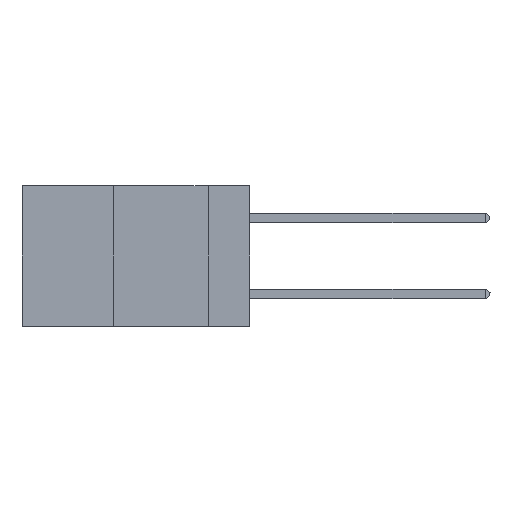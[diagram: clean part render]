
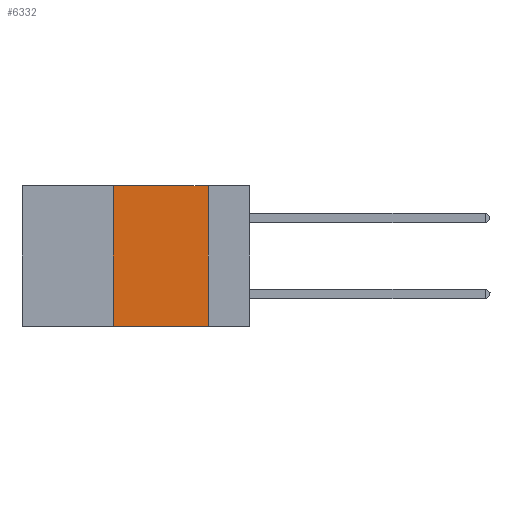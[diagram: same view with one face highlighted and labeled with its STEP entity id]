
A CAD part, left-side view. The second image highlights one B-rep face of the part: STEP entity #6332.
In plain terms, the highlighted planar face has unit normal (-1, 0, 0).
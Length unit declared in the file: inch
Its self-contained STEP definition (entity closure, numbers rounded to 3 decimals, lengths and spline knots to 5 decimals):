
#1540 = EDGE_CURVE ( 'NONE', #17693, #9061, #7145, .T. ) ;
#1716 = LINE ( 'NONE', #33998, #30821 ) ;
#2423 = VECTOR ( 'NONE', #25218, 39.37008 ) ;
#3049 = ORIENTED_EDGE ( 'NONE', *, *, #26859, .F. ) ;
#4459 = LINE ( 'NONE', #15882, #4602 ) ;
#4602 = VECTOR ( 'NONE', #21178, 39.37008 ) ;
#4839 = CARTESIAN_POINT ( 'NONE',  ( 0., 0.6, -0.37 ) ) ;
#5854 = CARTESIAN_POINT ( 'NONE',  ( 0., 0.6, 0. ) ) ;
#5883 = DIRECTION ( 'NONE',  ( 0., 0., -1. ) ) ;
#6332 = ADVANCED_FACE ( 'NONE', ( #7829 ), #34083, .F. ) ;
#7145 = LINE ( 'NONE', #4839, #18668 ) ;
#7829 = FACE_OUTER_BOUND ( 'NONE', #8242, .T. ) ;
#8237 = CARTESIAN_POINT ( 'NONE',  ( 0., 0.11, -0.37 ) ) ;
#8242 = EDGE_LOOP ( 'NONE', ( #3049, #34082, #18539, #13678 ) ) ;
#9061 = VERTEX_POINT ( 'NONE', #8237 ) ;
#10597 = AXIS2_PLACEMENT_3D ( 'NONE', #31429, #15391, #5883 ) ;
#12482 = DIRECTION ( 'NONE',  ( 0., 0., -1. ) ) ;
#13678 = ORIENTED_EDGE ( 'NONE', *, *, #1540, .T. ) ;
#15391 = DIRECTION ( 'NONE',  ( 1., 0., 0. ) ) ;
#15882 = CARTESIAN_POINT ( 'NONE',  ( 0., 0.36, 0. ) ) ;
#17554 = EDGE_CURVE ( 'NONE', #17693, #19803, #4459, .T. ) ;
#17693 = VERTEX_POINT ( 'NONE', #22048 ) ;
#18539 = ORIENTED_EDGE ( 'NONE', *, *, #17554, .F. ) ;
#18668 = VECTOR ( 'NONE', #20193, 39.37008 ) ;
#19595 = LINE ( 'NONE', #5854, #2423 ) ;
#19803 = VERTEX_POINT ( 'NONE', #27499 ) ;
#20193 = DIRECTION ( 'NONE',  ( 0., -1., 0. ) ) ;
#21047 = EDGE_CURVE ( 'NONE', #19803, #25376, #19595, .T. ) ;
#21178 = DIRECTION ( 'NONE',  ( 0., 0., 1. ) ) ;
#22048 = CARTESIAN_POINT ( 'NONE',  ( 0., 0.36, -0.37 ) ) ;
#25218 = DIRECTION ( 'NONE',  ( 0., -1., 0. ) ) ;
#25376 = VERTEX_POINT ( 'NONE', #30434 ) ;
#26859 = EDGE_CURVE ( 'NONE', #25376, #9061, #1716, .T. ) ;
#27499 = CARTESIAN_POINT ( 'NONE',  ( 0., 0.36, 0. ) ) ;
#30434 = CARTESIAN_POINT ( 'NONE',  ( 0., 0.11, 0. ) ) ;
#30821 = VECTOR ( 'NONE', #12482, 39.37008 ) ;
#31429 = CARTESIAN_POINT ( 'NONE',  ( 0., 0.6, 0. ) ) ;
#33998 = CARTESIAN_POINT ( 'NONE',  ( 0., 0.11, 0. ) ) ;
#34082 = ORIENTED_EDGE ( 'NONE', *, *, #21047, .F. ) ;
#34083 = PLANE ( 'NONE',  #10597 ) ;
